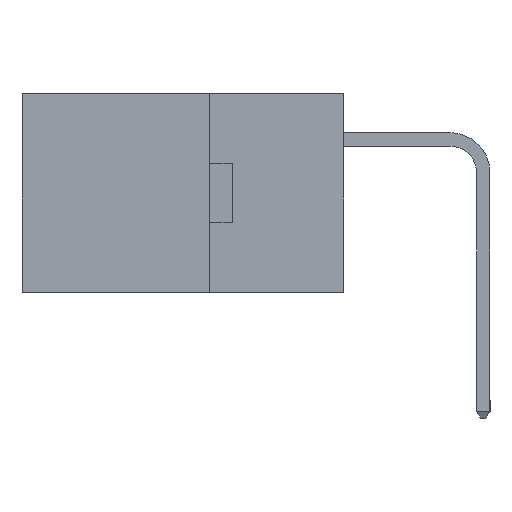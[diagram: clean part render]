
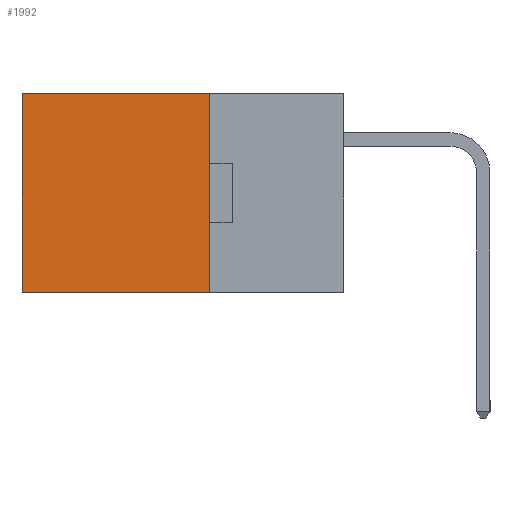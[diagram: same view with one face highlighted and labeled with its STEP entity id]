
A CAD part, left-side view. The second image highlights one B-rep face of the part: STEP entity #1992.
In plain terms, the highlighted planar face has unit normal (-1, 0, 0).
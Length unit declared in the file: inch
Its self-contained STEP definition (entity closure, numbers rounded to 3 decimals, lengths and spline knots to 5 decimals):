
#327 = DIRECTION ( 'NONE',  ( 0., 0., -1. ) ) ;
#407 = LINE ( 'NONE', #607, #10708 ) ;
#607 = CARTESIAN_POINT ( 'NONE',  ( 0.2615, 0.25, 0. ) ) ;
#1992 = ADVANCED_FACE ( 'NONE', ( #8212 ), #24900, .F. ) ;
#2220 = LINE ( 'NONE', #22875, #19267 ) ;
#3178 = CARTESIAN_POINT ( 'NONE',  ( 0.2615, 0.6, -0.37 ) ) ;
#3951 = EDGE_CURVE ( 'NONE', #20119, #14247, #407, .T. ) ;
#4752 = DIRECTION ( 'NONE',  ( 0., 0., -1. ) ) ;
#6443 = CARTESIAN_POINT ( 'NONE',  ( 0.2615, 0.25, 0. ) ) ;
#6701 = ORIENTED_EDGE ( 'NONE', *, *, #3951, .T. ) ;
#8212 = FACE_OUTER_BOUND ( 'NONE', #14593, .T. ) ;
#8280 = DIRECTION ( 'NONE',  ( 0., 1., 0. ) ) ;
#8994 = VECTOR ( 'NONE', #4752, 39.37008 ) ;
#10010 = CARTESIAN_POINT ( 'NONE',  ( 0.2615, 0.25, -0.37 ) ) ;
#10708 = VECTOR ( 'NONE', #12940, 39.37008 ) ;
#11206 = ORIENTED_EDGE ( 'NONE', *, *, #20197, .F. ) ;
#12655 = DIRECTION ( 'NONE',  ( 1., 0., 0. ) ) ;
#12656 = DIRECTION ( 'NONE',  ( 0., 0., -1. ) ) ;
#12940 = DIRECTION ( 'NONE',  ( 0., 1., 0. ) ) ;
#13721 = VECTOR ( 'NONE', #8280, 39.37008 ) ;
#14147 = VERTEX_POINT ( 'NONE', #3178 ) ;
#14247 = VERTEX_POINT ( 'NONE', #19742 ) ;
#14516 = EDGE_CURVE ( 'NONE', #16579, #14147, #24584, .T. ) ;
#14593 = EDGE_LOOP ( 'NONE', ( #19189, #17128, #11206, #6701 ) ) ;
#16579 = VERTEX_POINT ( 'NONE', #10010 ) ;
#16691 = AXIS2_PLACEMENT_3D ( 'NONE', #20824, #12655, #327 ) ;
#17128 = ORIENTED_EDGE ( 'NONE', *, *, #14516, .F. ) ;
#18581 = CARTESIAN_POINT ( 'NONE',  ( 0.2615, 0.25, -0.37 ) ) ;
#19189 = ORIENTED_EDGE ( 'NONE', *, *, #20709, .T. ) ;
#19267 = VECTOR ( 'NONE', #12656, 39.37008 ) ;
#19742 = CARTESIAN_POINT ( 'NONE',  ( 0.2615, 0.6, 0. ) ) ;
#20119 = VERTEX_POINT ( 'NONE', #6443 ) ;
#20197 = EDGE_CURVE ( 'NONE', #20119, #16579, #21850, .T. ) ;
#20709 = EDGE_CURVE ( 'NONE', #14247, #14147, #2220, .T. ) ;
#20824 = CARTESIAN_POINT ( 'NONE',  ( 0.2615, 0.25, -0.37 ) ) ;
#21850 = LINE ( 'NONE', #25192, #8994 ) ;
#22875 = CARTESIAN_POINT ( 'NONE',  ( 0.2615, 0.6, -0.37 ) ) ;
#24584 = LINE ( 'NONE', #18581, #13721 ) ;
#24900 = PLANE ( 'NONE',  #16691 ) ;
#25192 = CARTESIAN_POINT ( 'NONE',  ( 0.2615, 0.25, -0.37 ) ) ;
